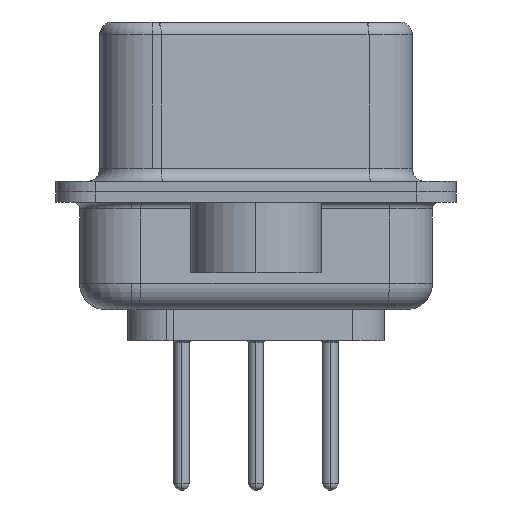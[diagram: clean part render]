
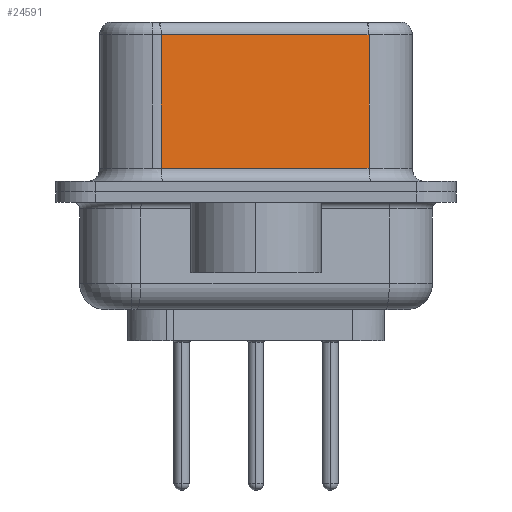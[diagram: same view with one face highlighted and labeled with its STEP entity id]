
A CAD part, left-side view. The second image highlights one B-rep face of the part: STEP entity #24591.
In plain terms, the highlighted planar face has unit normal (-0.985, -0.174, 0).
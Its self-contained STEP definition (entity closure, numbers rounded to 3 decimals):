
#317 = AXIS2_PLACEMENT_3D ( 'NONE', #24772, #13457, #22823 ) ;
#772 = LINE ( 'NONE', #9802, #23184 ) ;
#846 = VERTEX_POINT ( 'NONE', #2759 ) ;
#861 = ORIENTED_EDGE ( 'NONE', *, *, #26025, .T. ) ;
#1141 = DIRECTION ( 'NONE',  ( 0., 0., -1. ) ) ;
#1297 = EDGE_CURVE ( 'NONE', #26508, #27087, #13121, .T. ) ;
#1502 = VECTOR ( 'NONE', #1141, 1000. ) ;
#2759 = CARTESIAN_POINT ( 'NONE',  ( 3.73, 3.628, 0.9 ) ) ;
#6138 = DIRECTION ( 'NONE',  ( -0.174, 0.985, 0. ) ) ;
#6355 = CARTESIAN_POINT ( 'NONE',  ( 5.132, -4.322, 0.9 ) ) ;
#7843 = EDGE_CURVE ( 'NONE', #26508, #16340, #772, .T. ) ;
#8907 = CARTESIAN_POINT ( 'NONE',  ( 5.132, -4.322, 0.9 ) ) ;
#9802 = CARTESIAN_POINT ( 'NONE',  ( 5.132, -4.322, 6.52 ) ) ;
#9887 = LINE ( 'NONE', #18941, #1502 ) ;
#11336 = EDGE_CURVE ( 'NONE', #27087, #846, #9887, .T. ) ;
#12204 = CARTESIAN_POINT ( 'NONE',  ( 3.73, 3.628, 6.02 ) ) ;
#13121 = LINE ( 'NONE', #26477, #19022 ) ;
#13457 = DIRECTION ( 'NONE',  ( 0.985, 0.174, 0. ) ) ;
#13740 = ORIENTED_EDGE ( 'NONE', *, *, #11336, .T. ) ;
#14537 = DIRECTION ( 'NONE',  ( 0., 0., -1. ) ) ;
#15683 = PLANE ( 'NONE',  #317 ) ;
#16340 = VERTEX_POINT ( 'NONE', #6355 ) ;
#18019 = EDGE_LOOP ( 'NONE', ( #22750, #20305, #13740, #861 ) ) ;
#18353 = FACE_OUTER_BOUND ( 'NONE', #18019, .T. ) ;
#18941 = CARTESIAN_POINT ( 'NONE',  ( 3.73, 3.628, 6.52 ) ) ;
#19022 = VECTOR ( 'NONE', #6138, 1000. ) ;
#20305 = ORIENTED_EDGE ( 'NONE', *, *, #1297, .T. ) ;
#22750 = ORIENTED_EDGE ( 'NONE', *, *, #7843, .F. ) ;
#22823 = DIRECTION ( 'NONE',  ( -0.174, 0.985, 0. ) ) ;
#23184 = VECTOR ( 'NONE', #14537, 1000. ) ;
#24591 = ADVANCED_FACE ( 'NONE', ( #18353 ), #15683, .F. ) ;
#24657 = LINE ( 'NONE', #8907, #25994 ) ;
#24772 = CARTESIAN_POINT ( 'NONE',  ( 5.132, -4.322, 6.52 ) ) ;
#25994 = VECTOR ( 'NONE', #27145, 1000. ) ;
#26025 = EDGE_CURVE ( 'NONE', #846, #16340, #24657, .T. ) ;
#26477 = CARTESIAN_POINT ( 'NONE',  ( 5.132, -4.322, 6.02 ) ) ;
#26508 = VERTEX_POINT ( 'NONE', #26681 ) ;
#26681 = CARTESIAN_POINT ( 'NONE',  ( 5.132, -4.322, 6.02 ) ) ;
#27087 = VERTEX_POINT ( 'NONE', #12204 ) ;
#27145 = DIRECTION ( 'NONE',  ( 0.174, -0.985, 0. ) ) ;
